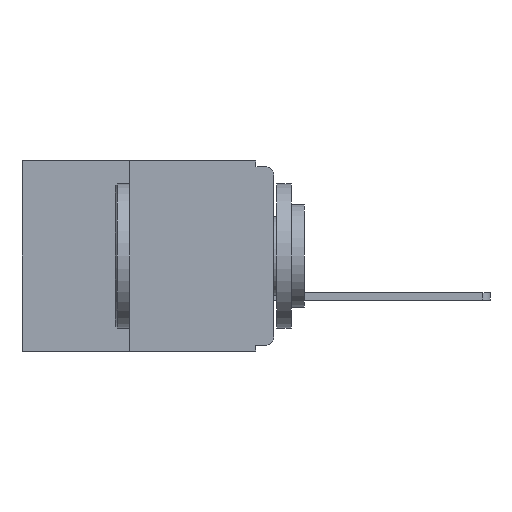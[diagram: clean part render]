
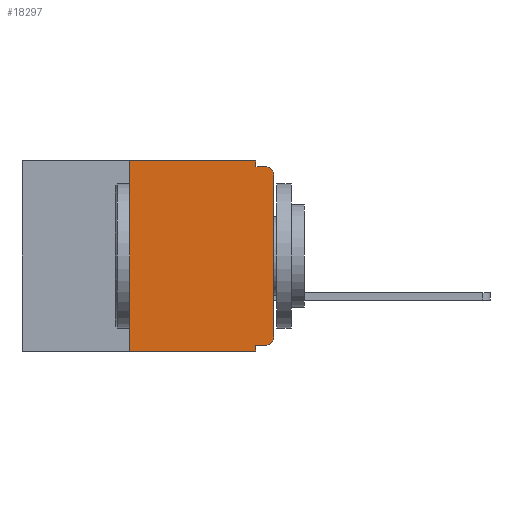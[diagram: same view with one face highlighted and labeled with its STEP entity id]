
A CAD part, left-side view. The second image highlights one B-rep face of the part: STEP entity #18297.
In plain terms, the highlighted planar face has unit normal (-1, 0, 0).
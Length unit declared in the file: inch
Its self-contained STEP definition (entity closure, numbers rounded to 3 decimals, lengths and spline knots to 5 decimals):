
#720 = DIRECTION ( 'NONE',  ( 0., -1., 0. ) ) ;
#1359 = LINE ( 'NONE', #4437, #21477 ) ;
#1688 = CARTESIAN_POINT ( 'NONE',  ( 0., 0., 0. ) ) ;
#1794 = LINE ( 'NONE', #22253, #16442 ) ;
#1941 = EDGE_CURVE ( 'NONE', #15813, #2915, #19454, .T. ) ;
#1980 = VERTEX_POINT ( 'NONE', #19860 ) ;
#2203 = EDGE_CURVE ( 'NONE', #10033, #1980, #9891, .T. ) ;
#2915 = VERTEX_POINT ( 'NONE', #6354 ) ;
#2955 = ORIENTED_EDGE ( 'NONE', *, *, #16209, .T. ) ;
#3028 = ORIENTED_EDGE ( 'NONE', *, *, #13457, .T. ) ;
#3180 = ORIENTED_EDGE ( 'NONE', *, *, #19760, .F. ) ;
#3251 = EDGE_CURVE ( 'NONE', #13818, #22258, #20554, .T. ) ;
#3294 = ORIENTED_EDGE ( 'NONE', *, *, #11932, .F. ) ;
#3383 = ORIENTED_EDGE ( 'NONE', *, *, #1941, .F. ) ;
#3463 = ORIENTED_EDGE ( 'NONE', *, *, #6963, .F. ) ;
#3486 = ORIENTED_EDGE ( 'NONE', *, *, #3251, .T. ) ;
#3689 = ORIENTED_EDGE ( 'NONE', *, *, #12929, .F. ) ;
#3697 = DIRECTION ( 'NONE',  ( 0., 0., 1. ) ) ;
#3789 = ORIENTED_EDGE ( 'NONE', *, *, #11060, .F. ) ;
#3929 = ORIENTED_EDGE ( 'NONE', *, *, #2203, .T. ) ;
#4123 = VECTOR ( 'NONE', #3697, 39.37008 ) ;
#4197 = LINE ( 'NONE', #7669, #8753 ) ;
#4437 = CARTESIAN_POINT ( 'NONE',  ( 0., 0., -0.01 ) ) ;
#4730 = VERTEX_POINT ( 'NONE', #19944 ) ;
#4814 = AXIS2_PLACEMENT_3D ( 'NONE', #16958, #5642, #18791 ) ;
#5021 = VERTEX_POINT ( 'NONE', #15063 ) ;
#5347 = CARTESIAN_POINT ( 'NONE',  ( 0., 0.437, 0. ) ) ;
#5642 = DIRECTION ( 'NONE',  ( -1., 0., 0. ) ) ;
#6354 = CARTESIAN_POINT ( 'NONE',  ( 0., 0.031, 0. ) ) ;
#6761 = VERTEX_POINT ( 'NONE', #14095 ) ;
#6963 = EDGE_CURVE ( 'NONE', #13818, #15813, #22787, .T. ) ;
#7195 = DIRECTION ( 'NONE',  ( 0., 0., 1. ) ) ;
#7409 = CARTESIAN_POINT ( 'NONE',  ( 0., 0.015, -0.305 ) ) ;
#7669 = CARTESIAN_POINT ( 'NONE',  ( 0., 0., -0.32 ) ) ;
#7897 = CARTESIAN_POINT ( 'NONE',  ( 0., 0.031, -0.33 ) ) ;
#7927 = VERTEX_POINT ( 'NONE', #17542 ) ;
#8272 = DIRECTION ( 'NONE',  ( 0., 0., -1. ) ) ;
#8288 = DIRECTION ( 'NONE',  ( -1., 0., 0. ) ) ;
#8705 = LINE ( 'NONE', #13638, #18008 ) ;
#8753 = VECTOR ( 'NONE', #18937, 39.37008 ) ;
#9281 = LINE ( 'NONE', #1688, #4123 ) ;
#9316 = DIRECTION ( 'NONE',  ( 0., 0., -1. ) ) ;
#9891 = CIRCLE ( 'NONE', #16656, 0.015 ) ;
#10033 = VERTEX_POINT ( 'NONE', #19604 ) ;
#11060 = EDGE_CURVE ( 'NONE', #10033, #7927, #4197, .T. ) ;
#11189 = DIRECTION ( 'NONE',  ( 0., 0., -1. ) ) ;
#11932 = EDGE_CURVE ( 'NONE', #2915, #5021, #8705, .T. ) ;
#12094 = DIRECTION ( 'NONE',  ( 0., -1., 0. ) ) ;
#12929 = EDGE_CURVE ( 'NONE', #7927, #22258, #1794, .T. ) ;
#13457 = EDGE_CURVE ( 'NONE', #6761, #4730, #15841, .T. ) ;
#13632 = VECTOR ( 'NONE', #7195, 39.37008 ) ;
#13638 = CARTESIAN_POINT ( 'NONE',  ( 0., 0.031, 0. ) ) ;
#13713 = DIRECTION ( 'NONE',  ( 0., 0., -1. ) ) ;
#13818 = VERTEX_POINT ( 'NONE', #19802 ) ;
#13913 = CARTESIAN_POINT ( 'NONE',  ( 0., 0.25, 0. ) ) ;
#14095 = CARTESIAN_POINT ( 'NONE',  ( 0., 0., -0.025 ) ) ;
#15063 = CARTESIAN_POINT ( 'NONE',  ( 0., 0.031, -0.01 ) ) ;
#15175 = VECTOR ( 'NONE', #22663, 39.37008 ) ;
#15670 = VECTOR ( 'NONE', #720, 39.37008 ) ;
#15813 = VERTEX_POINT ( 'NONE', #13913 ) ;
#15841 = CIRCLE ( 'NONE', #4814, 0.015 ) ;
#16209 = EDGE_CURVE ( 'NONE', #1980, #6761, #9281, .T. ) ;
#16442 = VECTOR ( 'NONE', #9316, 39.37008 ) ;
#16656 = AXIS2_PLACEMENT_3D ( 'NONE', #7409, #8288, #8272 ) ;
#16958 = CARTESIAN_POINT ( 'NONE',  ( 0., 0.015, -0.025 ) ) ;
#16986 = FACE_OUTER_BOUND ( 'NONE', #23046, .T. ) ;
#17542 = CARTESIAN_POINT ( 'NONE',  ( 0., 0.031, -0.32 ) ) ;
#18008 = VECTOR ( 'NONE', #13713, 39.37008 ) ;
#18297 = ADVANCED_FACE ( 'NONE', ( #16986 ), #18512, .F. ) ;
#18411 = CARTESIAN_POINT ( 'NONE',  ( 0., 0.25, -0.33 ) ) ;
#18512 = PLANE ( 'NONE',  #19517 ) ;
#18564 = CARTESIAN_POINT ( 'NONE',  ( 0., 0.437, -0.33 ) ) ;
#18791 = DIRECTION ( 'NONE',  ( 0., 0., -1. ) ) ;
#18937 = DIRECTION ( 'NONE',  ( 0., 1., 0. ) ) ;
#19454 = LINE ( 'NONE', #22693, #15175 ) ;
#19517 = AXIS2_PLACEMENT_3D ( 'NONE', #5347, #22195, #11189 ) ;
#19604 = CARTESIAN_POINT ( 'NONE',  ( 0., 0.015, -0.32 ) ) ;
#19760 = EDGE_CURVE ( 'NONE', #5021, #4730, #1359, .T. ) ;
#19802 = CARTESIAN_POINT ( 'NONE',  ( 0., 0.25, -0.33 ) ) ;
#19860 = CARTESIAN_POINT ( 'NONE',  ( 0., 0., -0.305 ) ) ;
#19944 = CARTESIAN_POINT ( 'NONE',  ( 0., 0.015, -0.01 ) ) ;
#20554 = LINE ( 'NONE', #18564, #15670 ) ;
#21477 = VECTOR ( 'NONE', #12094, 39.37008 ) ;
#22195 = DIRECTION ( 'NONE',  ( 1., 0., 0. ) ) ;
#22253 = CARTESIAN_POINT ( 'NONE',  ( 0., 0.031, -0.33 ) ) ;
#22258 = VERTEX_POINT ( 'NONE', #7897 ) ;
#22663 = DIRECTION ( 'NONE',  ( 0., -1., 0. ) ) ;
#22693 = CARTESIAN_POINT ( 'NONE',  ( 0., 0.437, 0. ) ) ;
#22787 = LINE ( 'NONE', #18411, #13632 ) ;
#23046 = EDGE_LOOP ( 'NONE', ( #2955, #3028, #3180, #3294, #3383, #3463, #3486, #3689, #3789, #3929 ) ) ;
